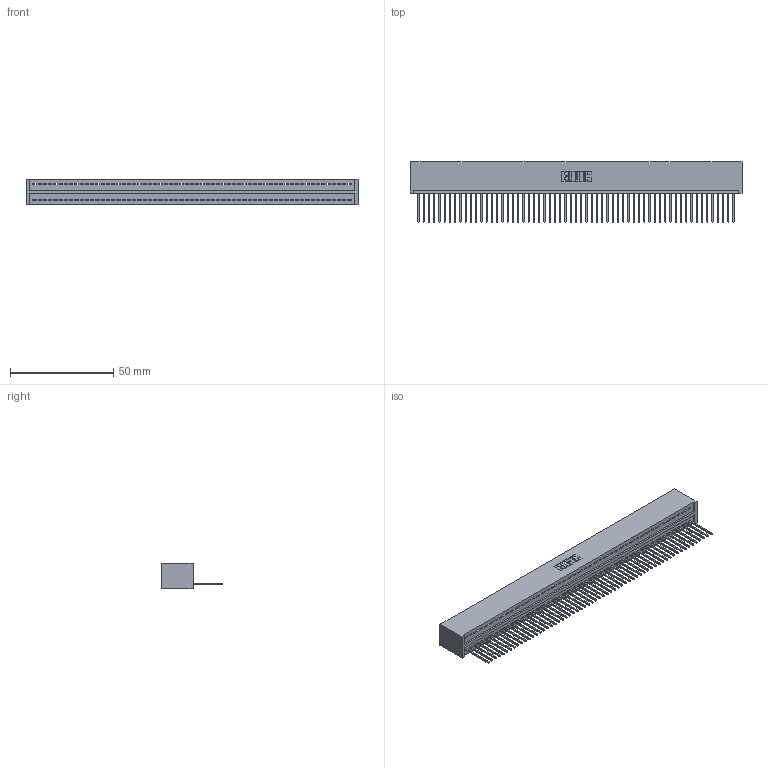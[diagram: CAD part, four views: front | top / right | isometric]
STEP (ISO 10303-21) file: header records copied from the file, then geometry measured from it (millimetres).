
FILE_DESCRIPTION (( 'STEP AP203' ), '1' );
FILE_NAME ('325-061-540-101.STEP', '2020-02-25T02:50:21', ( '' ), ( '' ), 'SwSTEP 2.0', 'SolidWorks 2016', '' );
FILE_SCHEMA (( 'CONFIG_CONTROL_DESIGN' ));
Length unit declared in the file: inch
Products named in the file (3): 325-292-001_325-293-140; 325 Part_Lugless; 325-061-540-101
Assembly tree (62 placements, depth 2):
  325-061-540-101
    325 Part_Lugless
    325-292-001_325-293-140  x61
Bounding box: 160.58 x 29.46 x 12.45 mm (x, y, z)
Volume: 21189.5 mm3; surface area: 24573.2 mm2
Topology: 62 solids, 62 shells, 3644 faces, 11023 edges, 7266 vertices
Faces by surface type: plane 2628, cylinder 1016
Entity records: 34575 total; most frequent: CARTESIAN_POINT 5969, ORIENTED_EDGE 5966, DIRECTION 4989, EDGE_CURVE 2983, VECTOR 2863, LINE 2863, VERTEX_POINT 1986, AXIS2_PLACEMENT_3D 1063
